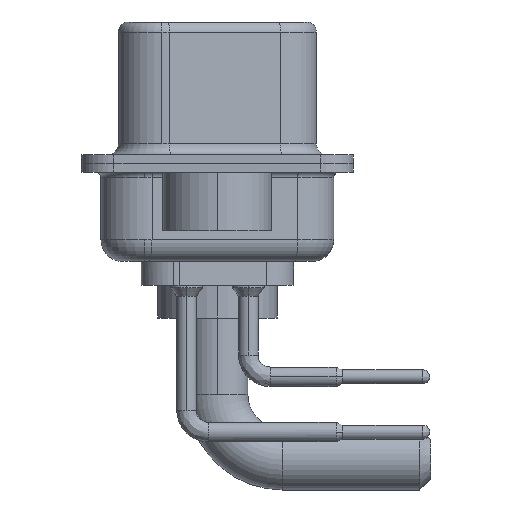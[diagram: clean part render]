
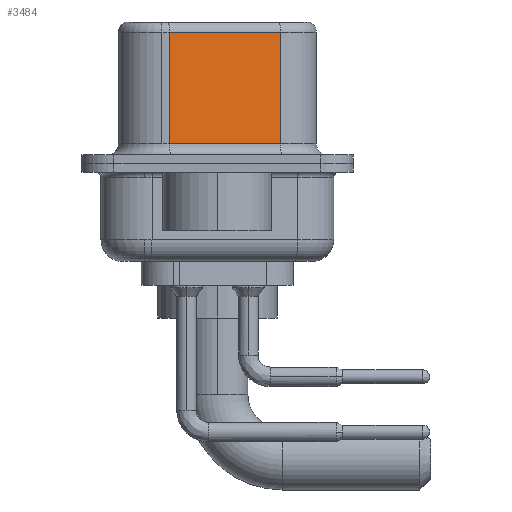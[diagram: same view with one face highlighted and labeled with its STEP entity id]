
A CAD part, left-side view. The second image highlights one B-rep face of the part: STEP entity #3484.
In plain terms, the highlighted planar face has unit normal (-0.985, -0.174, 0).
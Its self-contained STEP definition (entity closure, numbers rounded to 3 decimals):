
#1234 = CARTESIAN_POINT ( 'NONE',  ( 4.555, -2.897, 6.02 ) ) ;
#1855 = FACE_OUTER_BOUND ( 'NONE', #17384, .T. ) ;
#3294 = VECTOR ( 'NONE', #16331, 1000. ) ;
#3428 = CARTESIAN_POINT ( 'NONE',  ( 3.655, 2.203, 0.9 ) ) ;
#3484 = ADVANCED_FACE ( 'NONE', ( #1855 ), #12644, .F. ) ;
#3949 = CARTESIAN_POINT ( 'NONE',  ( 4.555, -2.897, 6.52 ) ) ;
#3992 = LINE ( 'NONE', #14663, #20522 ) ;
#4431 = AXIS2_PLACEMENT_3D ( 'NONE', #9004, #15940, #14225 ) ;
#4592 = CARTESIAN_POINT ( 'NONE',  ( 4.555, -2.897, 0.9 ) ) ;
#4932 = DIRECTION ( 'NONE',  ( 0.174, -0.985, 0. ) ) ;
#6620 = ORIENTED_EDGE ( 'NONE', *, *, #21785, .T. ) ;
#8274 = VERTEX_POINT ( 'NONE', #19440 ) ;
#8682 = VECTOR ( 'NONE', #4932, 1000. ) ;
#9004 = CARTESIAN_POINT ( 'NONE',  ( 4.555, -2.897, 6.52 ) ) ;
#9401 = LINE ( 'NONE', #13138, #3294 ) ;
#10902 = EDGE_CURVE ( 'NONE', #14340, #8274, #16414, .T. ) ;
#10997 = LINE ( 'NONE', #3949, #20916 ) ;
#12644 = PLANE ( 'NONE',  #4431 ) ;
#13138 = CARTESIAN_POINT ( 'NONE',  ( 4.555, -2.897, 6.02 ) ) ;
#13823 = ORIENTED_EDGE ( 'NONE', *, *, #10902, .T. ) ;
#14225 = DIRECTION ( 'NONE',  ( -0.174, 0.985, 0. ) ) ;
#14340 = VERTEX_POINT ( 'NONE', #3428 ) ;
#14663 = CARTESIAN_POINT ( 'NONE',  ( 3.655, 2.203, 6.52 ) ) ;
#14778 = DIRECTION ( 'NONE',  ( 0., 0., -1. ) ) ;
#15940 = DIRECTION ( 'NONE',  ( 0.985, 0.174, 0. ) ) ;
#15983 = ORIENTED_EDGE ( 'NONE', *, *, #16219, .T. ) ;
#16145 = ORIENTED_EDGE ( 'NONE', *, *, #18823, .F. ) ;
#16219 = EDGE_CURVE ( 'NONE', #21881, #14340, #3992, .T. ) ;
#16331 = DIRECTION ( 'NONE',  ( -0.174, 0.985, 0. ) ) ;
#16414 = LINE ( 'NONE', #4592, #8682 ) ;
#17384 = EDGE_LOOP ( 'NONE', ( #16145, #6620, #15983, #13823 ) ) ;
#17691 = DIRECTION ( 'NONE',  ( 0., 0., -1. ) ) ;
#18823 = EDGE_CURVE ( 'NONE', #21325, #8274, #10997, .T. ) ;
#19440 = CARTESIAN_POINT ( 'NONE',  ( 4.555, -2.897, 0.9 ) ) ;
#20398 = CARTESIAN_POINT ( 'NONE',  ( 3.655, 2.203, 6.02 ) ) ;
#20522 = VECTOR ( 'NONE', #14778, 1000. ) ;
#20916 = VECTOR ( 'NONE', #17691, 1000. ) ;
#21325 = VERTEX_POINT ( 'NONE', #1234 ) ;
#21785 = EDGE_CURVE ( 'NONE', #21325, #21881, #9401, .T. ) ;
#21881 = VERTEX_POINT ( 'NONE', #20398 ) ;
